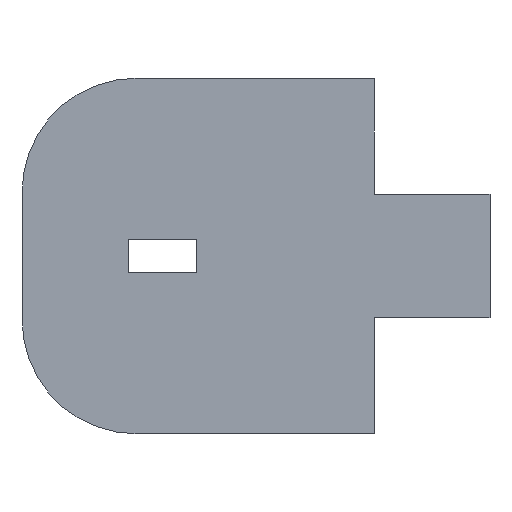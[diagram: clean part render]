
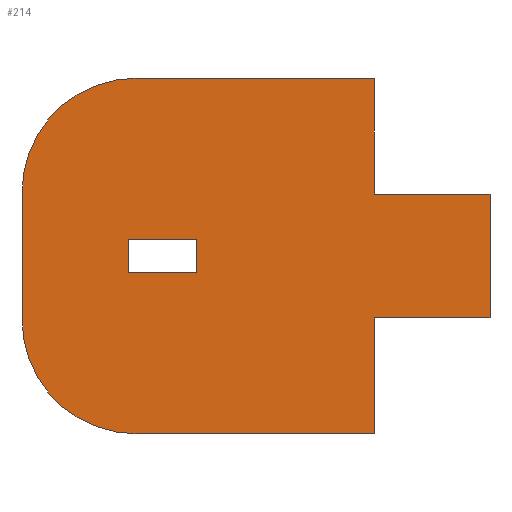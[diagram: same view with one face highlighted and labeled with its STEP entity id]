
A CAD part, left-side view. The second image highlights one B-rep face of the part: STEP entity #214.
In plain terms, the highlighted planar face has unit normal (-1, 0, 0).
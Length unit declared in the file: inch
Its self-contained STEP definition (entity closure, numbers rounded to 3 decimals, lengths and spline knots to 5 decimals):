
#6 = ORIENTED_EDGE ( 'NONE', *, *, #538, .F. ) ;
#8 = CARTESIAN_POINT ( 'NONE',  ( -0.08485, 0.19306, 0. ) ) ;
#13 = AXIS2_PLACEMENT_3D ( 'NONE', #634, #707, #191 ) ;
#19 = AXIS2_PLACEMENT_3D ( 'NONE', #93, #778, #244 ) ;
#28 = EDGE_CURVE ( 'NONE', #576, #706, #268, .T. ) ;
#30 = VERTEX_POINT ( 'NONE', #895 ) ;
#31 = DIRECTION ( 'NONE',  ( 0., 0., -1. ) ) ;
#42 = ORIENTED_EDGE ( 'NONE', *, *, #423, .T. ) ;
#56 = LINE ( 'NONE', #425, #430 ) ;
#71 = EDGE_LOOP ( 'NONE', ( #858, #168, #6, #42 ) ) ;
#93 = CARTESIAN_POINT ( 'NONE',  ( -0.08485, 1.02855, 0.43992 ) ) ;
#94 = VERTEX_POINT ( 'NONE', #684 ) ;
#106 = VECTOR ( 'NONE', #339, 39.37008 ) ;
#124 = LINE ( 'NONE', #315, #631 ) ;
#142 = ORIENTED_EDGE ( 'NONE', *, *, #928, .F. ) ;
#145 = EDGE_CURVE ( 'NONE', #811, #306, #302, .T. ) ;
#168 = ORIENTED_EDGE ( 'NONE', *, *, #145, .F. ) ;
#176 = DIRECTION ( 'NONE',  ( 0., 0., -1. ) ) ;
#179 = CARTESIAN_POINT ( 'NONE',  ( -0.08485, 0.19161, 0.43307 ) ) ;
#180 = VERTEX_POINT ( 'NONE', #692 ) ;
#191 = DIRECTION ( 'NONE',  ( 0., 0., 1. ) ) ;
#194 = CARTESIAN_POINT ( 'NONE',  ( -0.08485, 0., -0.40685 ) ) ;
#202 = LINE ( 'NONE', #271, #106 ) ;
#214 = ADVANCED_FACE ( 'NONE', ( #772, #364 ), #865, .T. ) ;
#219 = DIRECTION ( 'NONE',  ( 0., 0., -1. ) ) ;
#223 = ORIENTED_EDGE ( 'NONE', *, *, #936, .T. ) ;
#236 = CARTESIAN_POINT ( 'NONE',  ( -0.08485, 1.05666, 0. ) ) ;
#239 = CIRCLE ( 'NONE', #19, 0.4 ) ;
#244 = DIRECTION ( 'NONE',  ( 0., 0., 1. ) ) ;
#249 = ORIENTED_EDGE ( 'NONE', *, *, #807, .T. ) ;
#251 = DIRECTION ( 'NONE',  ( 0., 0., 1. ) ) ;
#252 = ORIENTED_EDGE ( 'NONE', *, *, #493, .T. ) ;
#268 = LINE ( 'NONE', #378, #432 ) ;
#271 = CARTESIAN_POINT ( 'NONE',  ( -0.08485, 0.93855, 0.62992 ) ) ;
#294 = CARTESIAN_POINT ( 'NONE',  ( -0.08485, -0.21245, 0. ) ) ;
#297 = EDGE_LOOP ( 'NONE', ( #782, #662, #249, #651, #223, #648, #443, #252, #609, #458, #626, #142 ) ) ;
#300 = VECTOR ( 'NONE', #176, 39.37008 ) ;
#301 = LINE ( 'NONE', #236, #722 ) ;
#302 = LINE ( 'NONE', #764, #690 ) ;
#306 = VERTEX_POINT ( 'NONE', #779 ) ;
#308 = VERTEX_POINT ( 'NONE', #179 ) ;
#311 = LINE ( 'NONE', #900, #536 ) ;
#315 = CARTESIAN_POINT ( 'NONE',  ( -0.08485, 1.42855, 0. ) ) ;
#320 = EDGE_CURVE ( 'NONE', #30, #308, #932, .T. ) ;
#336 = DIRECTION ( 'NONE',  ( 0., -1., 0. ) ) ;
#339 = DIRECTION ( 'NONE',  ( 0., -1., 0. ) ) ;
#364 = FACE_OUTER_BOUND ( 'NONE', #297, .T. ) ;
#376 = DIRECTION ( 'NONE',  ( -1., 0., 0. ) ) ;
#378 = CARTESIAN_POINT ( 'NONE',  ( -0.08485, 0.19306, 0. ) ) ;
#382 = VECTOR ( 'NONE', #667, 39.37008 ) ;
#407 = CARTESIAN_POINT ( 'NONE',  ( -0.08485, 0.19306, 0.62992 ) ) ;
#411 = VECTOR ( 'NONE', #716, 39.37008 ) ;
#415 = CARTESIAN_POINT ( 'NONE',  ( -0.08485, 0.19161, 0.62992 ) ) ;
#423 = EDGE_CURVE ( 'NONE', #602, #800, #931, .T. ) ;
#425 = CARTESIAN_POINT ( 'NONE',  ( -0.08485, 0., 0.83992 ) ) ;
#430 = VECTOR ( 'NONE', #653, 39.37008 ) ;
#432 = VECTOR ( 'NONE', #219, 39.37008 ) ;
#436 = CARTESIAN_POINT ( 'NONE',  ( -0.08485, 0.81666, 0. ) ) ;
#437 = EDGE_CURVE ( 'NONE', #94, #438, #56, .T. ) ;
#438 = VERTEX_POINT ( 'NONE', #647 ) ;
#443 = ORIENTED_EDGE ( 'NONE', *, *, #560, .F. ) ;
#450 = LINE ( 'NONE', #294, #515 ) ;
#457 = DIRECTION ( 'NONE',  ( 0., -1., 0. ) ) ;
#458 = ORIENTED_EDGE ( 'NONE', *, *, #320, .F. ) ;
#465 = VECTOR ( 'NONE', #660, 39.37008 ) ;
#467 = CARTESIAN_POINT ( 'NONE',  ( -0.08485, 1.42855, -0.00685 ) ) ;
#469 = DIRECTION ( 'NONE',  ( 0., 1., 0. ) ) ;
#476 = VERTEX_POINT ( 'NONE', #947 ) ;
#493 = EDGE_CURVE ( 'NONE', #615, #180, #580, .T. ) ;
#505 = AXIS2_PLACEMENT_3D ( 'NONE', #522, #376, #751 ) ;
#513 = CARTESIAN_POINT ( 'NONE',  ( -0.08485, 0.81666, 0.15748 ) ) ;
#515 = VECTOR ( 'NONE', #586, 39.37008 ) ;
#520 = CARTESIAN_POINT ( 'NONE',  ( -0.08485, -0.21245, -0.19685 ) ) ;
#522 = CARTESIAN_POINT ( 'NONE',  ( -0.08485, 1.02855, -0.00685 ) ) ;
#525 = CARTESIAN_POINT ( 'NONE',  ( -0.08485, 0.19306, -0.40685 ) ) ;
#536 = VECTOR ( 'NONE', #457, 39.37008 ) ;
#538 = EDGE_CURVE ( 'NONE', #602, #811, #723, .T. ) ;
#547 = CARTESIAN_POINT ( 'NONE',  ( -0.08485, 1.05666, 0.15748 ) ) ;
#560 = EDGE_CURVE ( 'NONE', #615, #576, #450, .T. ) ;
#564 = CARTESIAN_POINT ( 'NONE',  ( -0.08485, 1.02855, -0.40685 ) ) ;
#571 = CIRCLE ( 'NONE', #505, 0.4 ) ;
#576 = VERTEX_POINT ( 'NONE', #8 ) ;
#580 = LINE ( 'NONE', #520, #382 ) ;
#586 = DIRECTION ( 'NONE',  ( 0., 1., 0. ) ) ;
#602 = VERTEX_POINT ( 'NONE', #513 ) ;
#609 = ORIENTED_EDGE ( 'NONE', *, *, #705, .F. ) ;
#615 = VERTEX_POINT ( 'NONE', #743 ) ;
#623 = EDGE_CURVE ( 'NONE', #842, #924, #571, .T. ) ;
#626 = ORIENTED_EDGE ( 'NONE', *, *, #943, .F. ) ;
#631 = VECTOR ( 'NONE', #31, 39.37008 ) ;
#634 = CARTESIAN_POINT ( 'NONE',  ( -0.08485, 0.93855, -0.19685 ) ) ;
#647 = CARTESIAN_POINT ( 'NONE',  ( -0.08485, 0.19306, 0.83992 ) ) ;
#648 = ORIENTED_EDGE ( 'NONE', *, *, #28, .F. ) ;
#651 = ORIENTED_EDGE ( 'NONE', *, *, #623, .T. ) ;
#653 = DIRECTION ( 'NONE',  ( 0., -1., 0. ) ) ;
#660 = DIRECTION ( 'NONE',  ( 0., 0., 1. ) ) ;
#662 = ORIENTED_EDGE ( 'NONE', *, *, #823, .T. ) ;
#667 = DIRECTION ( 'NONE',  ( 0., 0., 1. ) ) ;
#684 = CARTESIAN_POINT ( 'NONE',  ( -0.08485, 1.02855, 0.83992 ) ) ;
#690 = VECTOR ( 'NONE', #469, 39.37008 ) ;
#692 = CARTESIAN_POINT ( 'NONE',  ( -0.08485, -0.21245, 0.43307 ) ) ;
#705 = EDGE_CURVE ( 'NONE', #308, #180, #311, .T. ) ;
#706 = VERTEX_POINT ( 'NONE', #525 ) ;
#707 = DIRECTION ( 'NONE',  ( -1., 0., 0. ) ) ;
#711 = LINE ( 'NONE', #713, #411 ) ;
#713 = CARTESIAN_POINT ( 'NONE',  ( -0.08485, 0.19306, 0. ) ) ;
#716 = DIRECTION ( 'NONE',  ( 0., 0., -1. ) ) ;
#722 = VECTOR ( 'NONE', #251, 39.37008 ) ;
#723 = LINE ( 'NONE', #436, #465 ) ;
#734 = VECTOR ( 'NONE', #950, 39.37008 ) ;
#743 = CARTESIAN_POINT ( 'NONE',  ( -0.08485, -0.21245, 0. ) ) ;
#744 = VERTEX_POINT ( 'NONE', #407 ) ;
#751 = DIRECTION ( 'NONE',  ( 0., 0., 1. ) ) ;
#764 = CARTESIAN_POINT ( 'NONE',  ( -0.08485, 0.55666, 0.27559 ) ) ;
#772 = FACE_BOUND ( 'NONE', #71, .T. ) ;
#777 = EDGE_CURVE ( 'NONE', #800, #306, #301, .T. ) ;
#778 = DIRECTION ( 'NONE',  ( -1., 0., 0. ) ) ;
#779 = CARTESIAN_POINT ( 'NONE',  ( -0.08485, 1.05666, 0.27559 ) ) ;
#782 = ORIENTED_EDGE ( 'NONE', *, *, #437, .F. ) ;
#800 = VERTEX_POINT ( 'NONE', #547 ) ;
#807 = EDGE_CURVE ( 'NONE', #476, #842, #124, .T. ) ;
#811 = VERTEX_POINT ( 'NONE', #835 ) ;
#823 = EDGE_CURVE ( 'NONE', #94, #476, #239, .T. ) ;
#825 = LINE ( 'NONE', #194, #836 ) ;
#835 = CARTESIAN_POINT ( 'NONE',  ( -0.08485, 0.81666, 0.27559 ) ) ;
#836 = VECTOR ( 'NONE', #336, 39.37008 ) ;
#842 = VERTEX_POINT ( 'NONE', #467 ) ;
#858 = ORIENTED_EDGE ( 'NONE', *, *, #777, .T. ) ;
#865 = PLANE ( 'NONE',  #13 ) ;
#877 = CARTESIAN_POINT ( 'NONE',  ( -0.08485, 0., 0.15748 ) ) ;
#895 = CARTESIAN_POINT ( 'NONE',  ( -0.08485, 0.19161, 0.62992 ) ) ;
#900 = CARTESIAN_POINT ( 'NONE',  ( -0.08485, 0.19161, 0.43307 ) ) ;
#924 = VERTEX_POINT ( 'NONE', #564 ) ;
#928 = EDGE_CURVE ( 'NONE', #438, #744, #711, .T. ) ;
#931 = LINE ( 'NONE', #877, #734 ) ;
#932 = LINE ( 'NONE', #415, #300 ) ;
#936 = EDGE_CURVE ( 'NONE', #924, #706, #825, .T. ) ;
#943 = EDGE_CURVE ( 'NONE', #744, #30, #202, .T. ) ;
#947 = CARTESIAN_POINT ( 'NONE',  ( -0.08485, 1.42855, 0.43992 ) ) ;
#950 = DIRECTION ( 'NONE',  ( 0., 1., 0. ) ) ;
